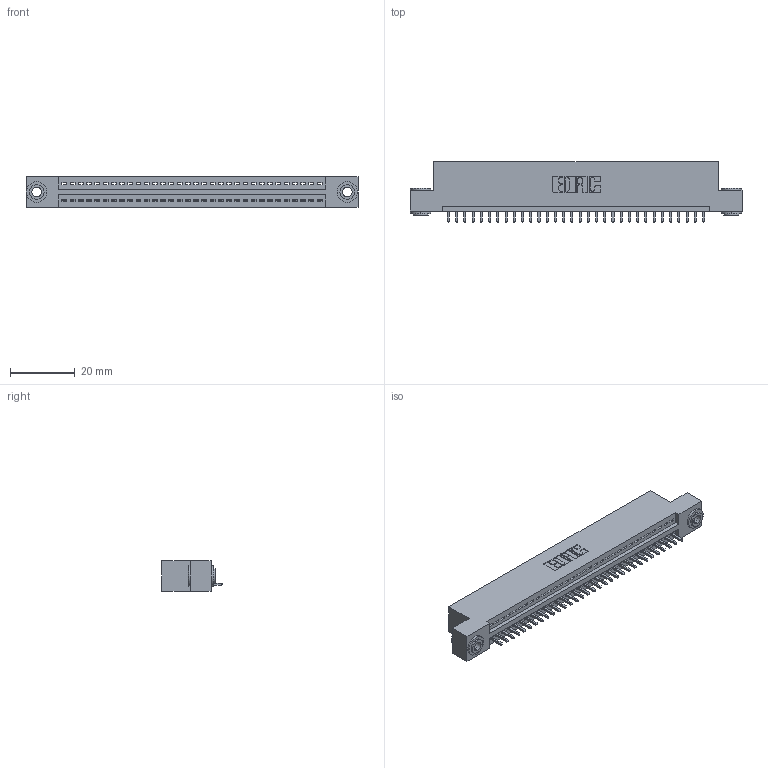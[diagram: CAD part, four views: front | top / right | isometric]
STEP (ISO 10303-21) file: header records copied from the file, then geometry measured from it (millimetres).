
FILE_DESCRIPTION (( 'STEP AP203' ), '1' );
FILE_NAME ('395-032-521-103.STEP', '2019-10-19T13:50:19', ( '' ), ( '' ), 'SwSTEP 2.0', 'SolidWorks 2016', '' );
FILE_SCHEMA (( 'CONFIG_CONTROL_DESIGN' ));
Length unit declared in the file: inch
Products named in the file (4): 345-250-002_345-250-002-102; 395-032-521-103; 345-292-001_345-293-121; 345 Part_Flush Mounting Lugs - 0.156 Dia-TH
Assembly tree (35 placements, depth 2):
  395-032-521-103
    345 Part_Flush Mounting Lugs - 0.156 Dia-TH
    345-292-001_345-293-121  x32
    345-250-002_345-250-002-102  x2
Bounding box: 102.49 x 18.72 x 9.4 mm (x, y, z)
Volume: 9580.9 mm3; surface area: 12454.7 mm2
Topology: 35 solids, 35 shells, 2020 faces, 6049 edges, 3986 vertices
Faces by surface type: plane 1370, cylinder 642, cone 8
Entity records: 26098 total; most frequent: CARTESIAN_POINT 4499, ORIENTED_EDGE 4458, DIRECTION 3975, EDGE_CURVE 2229, LINE 1945, VECTOR 1945, VERTEX_POINT 1482, AXIS2_PLACEMENT_3D 1015
